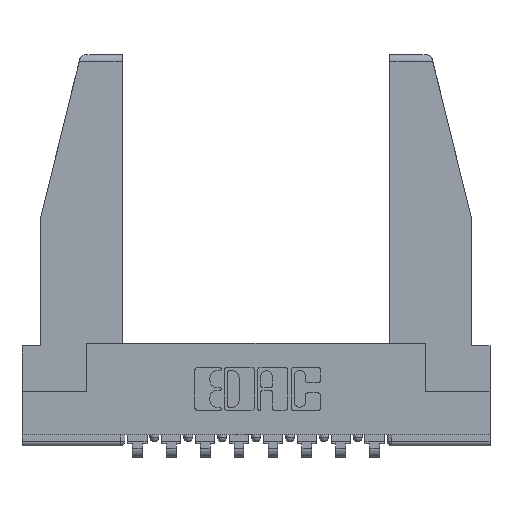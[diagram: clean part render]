
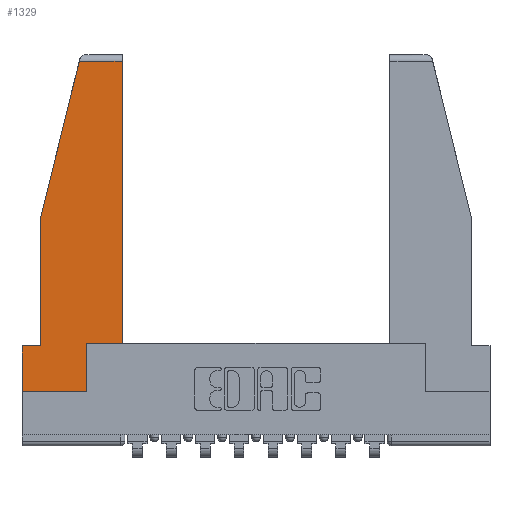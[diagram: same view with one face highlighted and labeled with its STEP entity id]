
A CAD part, top view. The second image highlights one B-rep face of the part: STEP entity #1329.
In plain terms, the highlighted planar face has unit normal (0, 0, 1).
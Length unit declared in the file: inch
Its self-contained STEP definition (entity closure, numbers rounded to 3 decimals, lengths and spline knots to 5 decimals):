
#622 = CARTESIAN_POINT ( 'NONE',  ( 0.297, 0., 0. ) ) ;
#783 = ORIENTED_EDGE ( 'NONE', *, *, #10191, .T. ) ;
#833 = EDGE_CURVE ( 'NONE', #8942, #6047, #12072, .T. ) ;
#850 = DIRECTION ( 'NONE',  ( -0.239, -0.971, 0. ) ) ;
#922 = CARTESIAN_POINT ( 'NONE',  ( 0., 0., 0. ) ) ;
#979 = CARTESIAN_POINT ( 'NONE',  ( 0.086, 0.8, 0. ) ) ;
#1069 = EDGE_CURVE ( 'NONE', #5648, #5385, #8406, .T. ) ;
#1133 = DIRECTION ( 'NONE',  ( 0., 1., 0. ) ) ;
#1329 = ADVANCED_FACE ( 'NONE', ( #12405 ), #8218, .T. ) ;
#1374 = VERTEX_POINT ( 'NONE', #8315 ) ;
#1500 = EDGE_CURVE ( 'NONE', #9251, #4781, #9256, .T. ) ;
#1567 = EDGE_CURVE ( 'NONE', #6047, #9251, #10999, .T. ) ;
#1598 = DIRECTION ( 'NONE',  ( 0., 0., 1. ) ) ;
#2033 = DIRECTION ( 'NONE',  ( 1., 0., 0. ) ) ;
#2231 = CARTESIAN_POINT ( 'NONE',  ( 0., 0.21, 0. ) ) ;
#2999 = VECTOR ( 'NONE', #7403, 39.37008 ) ;
#3320 = CARTESIAN_POINT ( 'NONE',  ( 0., 0.21, 0. ) ) ;
#3688 = VECTOR ( 'NONE', #4080, 39.37008 ) ;
#3893 = VECTOR ( 'NONE', #10308, 39.37008 ) ;
#3954 = VECTOR ( 'NONE', #7487, 39.37008 ) ;
#4080 = DIRECTION ( 'NONE',  ( 0., 1., 0. ) ) ;
#4613 = EDGE_CURVE ( 'NONE', #1374, #10333, #6400, .T. ) ;
#4781 = VERTEX_POINT ( 'NONE', #10128 ) ;
#5030 = ORIENTED_EDGE ( 'NONE', *, *, #1069, .T. ) ;
#5153 = EDGE_CURVE ( 'NONE', #4781, #5648, #6560, .T. ) ;
#5385 = VERTEX_POINT ( 'NONE', #7770 ) ;
#5393 = EDGE_CURVE ( 'NONE', #7895, #8942, #14348, .T. ) ;
#5587 = EDGE_LOOP ( 'NONE', ( #5030, #8021, #12417, #783, #10787, #5952, #14364, #7380, #6149 ) ) ;
#5648 = VERTEX_POINT ( 'NONE', #10441 ) ;
#5952 = ORIENTED_EDGE ( 'NONE', *, *, #833, .T. ) ;
#6047 = VERTEX_POINT ( 'NONE', #9179 ) ;
#6149 = ORIENTED_EDGE ( 'NONE', *, *, #5153, .T. ) ;
#6386 = CARTESIAN_POINT ( 'NONE',  ( 0.271, 1.55, 0. ) ) ;
#6400 = LINE ( 'NONE', #6386, #13842 ) ;
#6560 = LINE ( 'NONE', #8386, #3954 ) ;
#7209 = VECTOR ( 'NONE', #8662, 39.37008 ) ;
#7242 = VECTOR ( 'NONE', #11083, 39.37008 ) ;
#7380 = ORIENTED_EDGE ( 'NONE', *, *, #1500, .T. ) ;
#7403 = DIRECTION ( 'NONE',  ( 0., -1., 0. ) ) ;
#7487 = DIRECTION ( 'NONE',  ( 1., 0., 0. ) ) ;
#7770 = CARTESIAN_POINT ( 'NONE',  ( 0.461, 1.52, 0. ) ) ;
#7856 = VECTOR ( 'NONE', #2033, 39.37008 ) ;
#7895 = VERTEX_POINT ( 'NONE', #9443 ) ;
#8021 = ORIENTED_EDGE ( 'NONE', *, *, #14360, .T. ) ;
#8218 = PLANE ( 'NONE',  #11142 ) ;
#8315 = CARTESIAN_POINT ( 'NONE',  ( 0.2636, 1.52, 0. ) ) ;
#8386 = CARTESIAN_POINT ( 'NONE',  ( 0.297, 0.223, 0. ) ) ;
#8406 = LINE ( 'NONE', #13354, #9625 ) ;
#8662 = DIRECTION ( 'NONE',  ( 0., -1., 0. ) ) ;
#8942 = VERTEX_POINT ( 'NONE', #3320 ) ;
#9179 = CARTESIAN_POINT ( 'NONE',  ( 0., 0., 0. ) ) ;
#9251 = VERTEX_POINT ( 'NONE', #622 ) ;
#9256 = LINE ( 'NONE', #10649, #3688 ) ;
#9434 = CARTESIAN_POINT ( 'NONE',  ( 0., 0., 0. ) ) ;
#9443 = CARTESIAN_POINT ( 'NONE',  ( 0.086, 0.21, 0. ) ) ;
#9574 = CARTESIAN_POINT ( 'NONE',  ( 0.086, 0.8, 0. ) ) ;
#9625 = VECTOR ( 'NONE', #1133, 39.37008 ) ;
#10128 = CARTESIAN_POINT ( 'NONE',  ( 0.297, 0.223, 0. ) ) ;
#10191 = EDGE_CURVE ( 'NONE', #10333, #7895, #11343, .T. ) ;
#10308 = DIRECTION ( 'NONE',  ( -1., 0., 0. ) ) ;
#10333 = VERTEX_POINT ( 'NONE', #979 ) ;
#10441 = CARTESIAN_POINT ( 'NONE',  ( 0.461, 0.223, 0. ) ) ;
#10504 = LINE ( 'NONE', #10595, #3893 ) ;
#10595 = CARTESIAN_POINT ( 'NONE',  ( 0., 1.52, 0. ) ) ;
#10649 = CARTESIAN_POINT ( 'NONE',  ( 0.297, 0., 0. ) ) ;
#10787 = ORIENTED_EDGE ( 'NONE', *, *, #5393, .T. ) ;
#10898 = CARTESIAN_POINT ( 'NONE',  ( 0., 0.21, 0. ) ) ;
#10999 = LINE ( 'NONE', #922, #7856 ) ;
#11083 = DIRECTION ( 'NONE',  ( -1., 0., 0. ) ) ;
#11142 = AXIS2_PLACEMENT_3D ( 'NONE', #9434, #1598, #13815 ) ;
#11343 = LINE ( 'NONE', #9574, #2999 ) ;
#12072 = LINE ( 'NONE', #10898, #7209 ) ;
#12405 = FACE_OUTER_BOUND ( 'NONE', #5587, .T. ) ;
#12417 = ORIENTED_EDGE ( 'NONE', *, *, #4613, .T. ) ;
#13354 = CARTESIAN_POINT ( 'NONE',  ( 0.461, 0.223, 0. ) ) ;
#13815 = DIRECTION ( 'NONE',  ( 1., 0., 0. ) ) ;
#13842 = VECTOR ( 'NONE', #850, 39.37008 ) ;
#14348 = LINE ( 'NONE', #2231, #7242 ) ;
#14360 = EDGE_CURVE ( 'NONE', #5385, #1374, #10504, .T. ) ;
#14364 = ORIENTED_EDGE ( 'NONE', *, *, #1567, .T. ) ;
